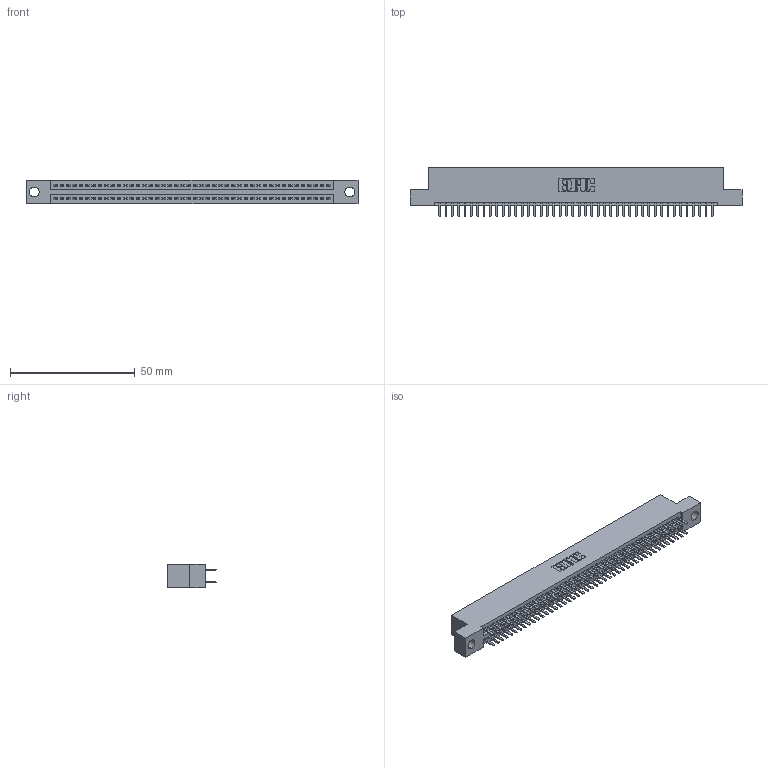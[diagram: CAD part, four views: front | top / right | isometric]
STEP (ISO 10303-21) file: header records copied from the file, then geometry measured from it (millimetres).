
FILE_DESCRIPTION (( 'STEP AP203' ), '1' );
FILE_NAME ('395-088-520-204.STEP', '2021-06-17T09:16:03', ( '' ), ( '' ), 'SwSTEP 2.0', 'SolidWorks 2020', '' );
FILE_SCHEMA (( 'CONFIG_CONTROL_DESIGN' ));
Length unit declared in the file: inch
Products named in the file (3): 395-088-520-204; 345-292-001_345-293-120; 345 Part_Flush Mounting Lugs - 0.156 Dia-TI
Assembly tree (89 placements, depth 2):
  395-088-520-204
    345 Part_Flush Mounting Lugs - 0.156 Dia-TI
    345-292-001_345-293-120  x88
Bounding box: 132.97 x 19.68 x 9.4 mm (x, y, z)
Volume: 12790.7 mm3; surface area: 18714.8 mm2
Topology: 89 solids, 89 shells, 4892 faces, 14193 edges, 9226 vertices
Faces by surface type: plane 3174, cylinder 1718
Entity records: 34787 total; most frequent: CARTESIAN_POINT 5846, ORIENTED_EDGE 5766, DIRECTION 5139, EDGE_CURVE 2883, VECTOR 2571, LINE 2571, VERTEX_POINT 1918, AXIS2_PLACEMENT_3D 1284
